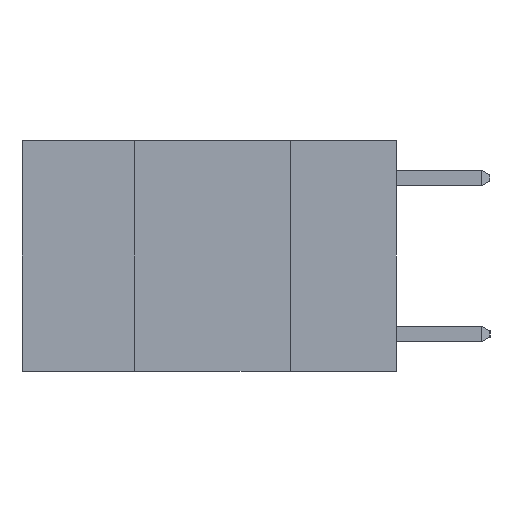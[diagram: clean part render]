
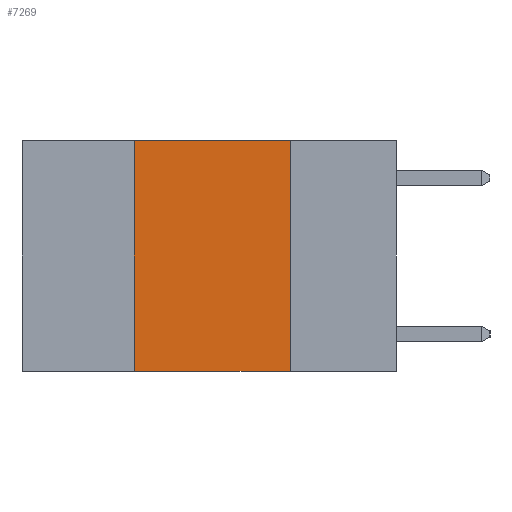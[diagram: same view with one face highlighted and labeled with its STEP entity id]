
A CAD part, left-side view. The second image highlights one B-rep face of the part: STEP entity #7269.
In plain terms, the highlighted planar face has unit normal (-1, 0, 0).
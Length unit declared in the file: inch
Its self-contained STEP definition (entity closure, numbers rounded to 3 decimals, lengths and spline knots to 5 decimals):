
#99 = VERTEX_POINT ( 'NONE', #11499 ) ;
#300 = CARTESIAN_POINT ( 'NONE',  ( 0., 0.17, -0.37 ) ) ;
#537 = CARTESIAN_POINT ( 'NONE',  ( 0., 0.6, -0.37 ) ) ;
#584 = ORIENTED_EDGE ( 'NONE', *, *, #3513, .T. ) ;
#657 = EDGE_CURVE ( 'NONE', #99, #10677, #7617, .T. ) ;
#1455 = DIRECTION ( 'NONE',  ( 0., -1., 0. ) ) ;
#1495 = PLANE ( 'NONE',  #11433 ) ;
#1538 = CARTESIAN_POINT ( 'NONE',  ( 0., 0.6, 0. ) ) ;
#1544 = VECTOR ( 'NONE', #10090, 39.37008 ) ;
#1609 = LINE ( 'NONE', #10917, #6196 ) ;
#2157 = VECTOR ( 'NONE', #3559, 39.37008 ) ;
#2760 = CARTESIAN_POINT ( 'NONE',  ( 0., 0.17, 0. ) ) ;
#3381 = DIRECTION ( 'NONE',  ( 0., 0., -1. ) ) ;
#3513 = EDGE_CURVE ( 'NONE', #9664, #5259, #6982, .T. ) ;
#3559 = DIRECTION ( 'NONE',  ( 0., -1., 0. ) ) ;
#3783 = CARTESIAN_POINT ( 'NONE',  ( 0., 0.17, 0. ) ) ;
#4269 = LINE ( 'NONE', #2760, #1544 ) ;
#4367 = ORIENTED_EDGE ( 'NONE', *, *, #9875, .F. ) ;
#4543 = VECTOR ( 'NONE', #1455, 39.37008 ) ;
#5259 = VERTEX_POINT ( 'NONE', #300 ) ;
#5736 = EDGE_LOOP ( 'NONE', ( #9200, #6990, #4367, #584 ) ) ;
#6196 = VECTOR ( 'NONE', #6321, 39.37008 ) ;
#6273 = EDGE_CURVE ( 'NONE', #10677, #5259, #4269, .T. ) ;
#6284 = CARTESIAN_POINT ( 'NONE',  ( 0., 0.6, 0. ) ) ;
#6321 = DIRECTION ( 'NONE',  ( 0., 0., 1. ) ) ;
#6982 = LINE ( 'NONE', #537, #4543 ) ;
#6990 = ORIENTED_EDGE ( 'NONE', *, *, #657, .F. ) ;
#7269 = ADVANCED_FACE ( 'NONE', ( #8110 ), #1495, .F. ) ;
#7617 = LINE ( 'NONE', #6284, #2157 ) ;
#8110 = FACE_OUTER_BOUND ( 'NONE', #5736, .T. ) ;
#8789 = CARTESIAN_POINT ( 'NONE',  ( 0., 0.42, -0.37 ) ) ;
#8882 = DIRECTION ( 'NONE',  ( 1., 0., 0. ) ) ;
#9200 = ORIENTED_EDGE ( 'NONE', *, *, #6273, .F. ) ;
#9664 = VERTEX_POINT ( 'NONE', #8789 ) ;
#9875 = EDGE_CURVE ( 'NONE', #9664, #99, #1609, .T. ) ;
#10090 = DIRECTION ( 'NONE',  ( 0., 0., -1. ) ) ;
#10677 = VERTEX_POINT ( 'NONE', #3783 ) ;
#10917 = CARTESIAN_POINT ( 'NONE',  ( 0., 0.42, 0. ) ) ;
#11433 = AXIS2_PLACEMENT_3D ( 'NONE', #1538, #8882, #3381 ) ;
#11499 = CARTESIAN_POINT ( 'NONE',  ( 0., 0.42, 0. ) ) ;
